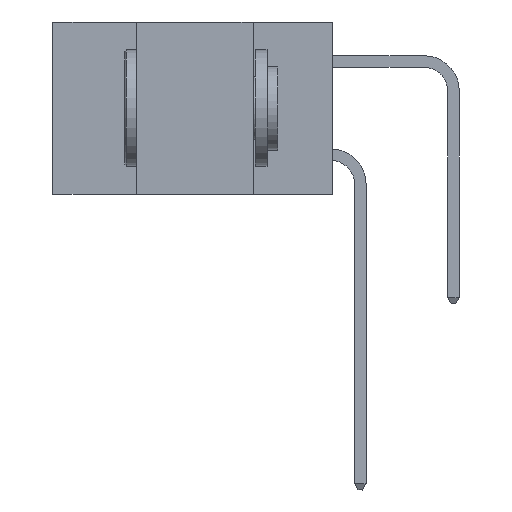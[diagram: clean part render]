
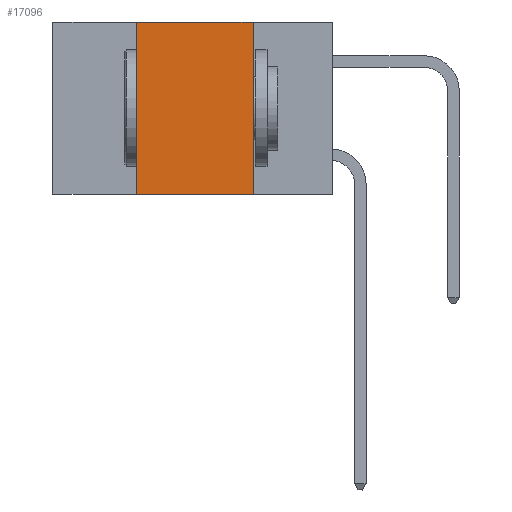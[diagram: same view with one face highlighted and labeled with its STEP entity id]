
A CAD part, left-side view. The second image highlights one B-rep face of the part: STEP entity #17096.
In plain terms, the highlighted planar face has unit normal (-1, 0, 0).
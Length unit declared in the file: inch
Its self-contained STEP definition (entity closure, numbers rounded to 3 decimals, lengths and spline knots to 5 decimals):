
#641 = ORIENTED_EDGE ( 'NONE', *, *, #2065, .F. ) ;
#717 = CARTESIAN_POINT ( 'NONE',  ( 0., 0.42, 0. ) ) ;
#1482 = CARTESIAN_POINT ( 'NONE',  ( 0., 0.42, 0. ) ) ;
#2065 = EDGE_CURVE ( 'NONE', #4525, #10353, #4750, .T. ) ;
#2196 = CARTESIAN_POINT ( 'NONE',  ( 0., 0.17, 0. ) ) ;
#2499 = DIRECTION ( 'NONE',  ( 0., -1., 0. ) ) ;
#2798 = LINE ( 'NONE', #1482, #3454 ) ;
#2837 = CARTESIAN_POINT ( 'NONE',  ( 0., 0.17, 0. ) ) ;
#2899 = CARTESIAN_POINT ( 'NONE',  ( 0., 0.6, 0. ) ) ;
#3244 = CARTESIAN_POINT ( 'NONE',  ( 0., 0.6, 0. ) ) ;
#3454 = VECTOR ( 'NONE', #15194, 39.37008 ) ;
#4453 = DIRECTION ( 'NONE',  ( 0., 0., -1. ) ) ;
#4525 = VERTEX_POINT ( 'NONE', #2837 ) ;
#4598 = DIRECTION ( 'NONE',  ( 0., -1., 0. ) ) ;
#4750 = LINE ( 'NONE', #2196, #9059 ) ;
#4826 = LINE ( 'NONE', #3244, #15333 ) ;
#6408 = VERTEX_POINT ( 'NONE', #717 ) ;
#6921 = CARTESIAN_POINT ( 'NONE',  ( 0., 0.42, -0.37 ) ) ;
#6997 = VECTOR ( 'NONE', #2499, 39.37008 ) ;
#8939 = FACE_OUTER_BOUND ( 'NONE', #9068, .T. ) ;
#9059 = VECTOR ( 'NONE', #14649, 39.37008 ) ;
#9068 = EDGE_LOOP ( 'NONE', ( #641, #15846, #16685, #16073 ) ) ;
#10353 = VERTEX_POINT ( 'NONE', #13789 ) ;
#12865 = EDGE_CURVE ( 'NONE', #12981, #10353, #13009, .T. ) ;
#12981 = VERTEX_POINT ( 'NONE', #6921 ) ;
#13009 = LINE ( 'NONE', #16097, #6997 ) ;
#13789 = CARTESIAN_POINT ( 'NONE',  ( 0., 0.17, -0.37 ) ) ;
#14649 = DIRECTION ( 'NONE',  ( 0., 0., -1. ) ) ;
#15194 = DIRECTION ( 'NONE',  ( 0., 0., 1. ) ) ;
#15227 = EDGE_CURVE ( 'NONE', #12981, #6408, #2798, .T. ) ;
#15333 = VECTOR ( 'NONE', #4598, 39.37008 ) ;
#15363 = DIRECTION ( 'NONE',  ( 1., 0., 0. ) ) ;
#15761 = AXIS2_PLACEMENT_3D ( 'NONE', #2899, #15363, #4453 ) ;
#15846 = ORIENTED_EDGE ( 'NONE', *, *, #17702, .F. ) ;
#16073 = ORIENTED_EDGE ( 'NONE', *, *, #12865, .T. ) ;
#16097 = CARTESIAN_POINT ( 'NONE',  ( 0., 0.6, -0.37 ) ) ;
#16685 = ORIENTED_EDGE ( 'NONE', *, *, #15227, .F. ) ;
#16786 = PLANE ( 'NONE',  #15761 ) ;
#17096 = ADVANCED_FACE ( 'NONE', ( #8939 ), #16786, .F. ) ;
#17702 = EDGE_CURVE ( 'NONE', #6408, #4525, #4826, .T. ) ;
